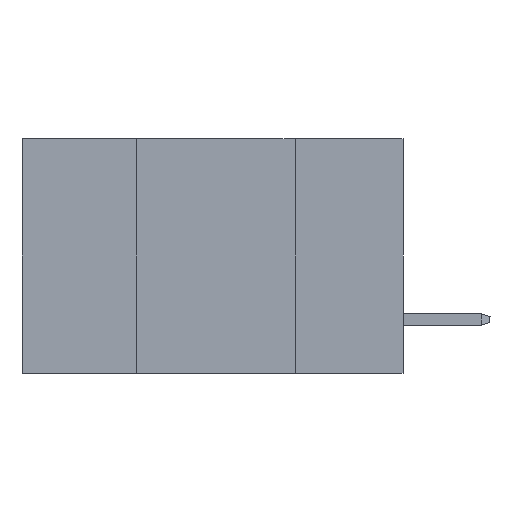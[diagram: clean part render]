
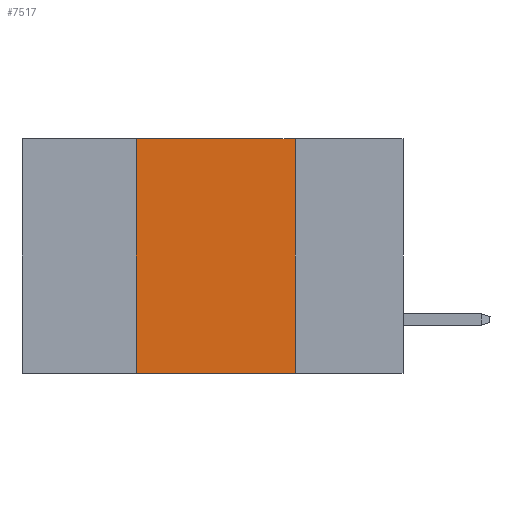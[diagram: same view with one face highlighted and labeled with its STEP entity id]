
A CAD part, left-side view. The second image highlights one B-rep face of the part: STEP entity #7517.
In plain terms, the highlighted planar face has unit normal (-1, 0, 0).
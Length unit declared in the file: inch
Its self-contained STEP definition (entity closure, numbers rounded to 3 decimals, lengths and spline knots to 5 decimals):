
#582 = CARTESIAN_POINT ( 'NONE',  ( 0., 0.6, 0. ) ) ;
#982 = LINE ( 'NONE', #5002, #21636 ) ;
#1261 = CARTESIAN_POINT ( 'NONE',  ( 0., 0.17, 0. ) ) ;
#1351 = VERTEX_POINT ( 'NONE', #9151 ) ;
#1695 = AXIS2_PLACEMENT_3D ( 'NONE', #582, #12738, #18744 ) ;
#3512 = ORIENTED_EDGE ( 'NONE', *, *, #24849, .T. ) ;
#4922 = LINE ( 'NONE', #15397, #11618 ) ;
#5002 = CARTESIAN_POINT ( 'NONE',  ( 0., 0.42, 0. ) ) ;
#6378 = VERTEX_POINT ( 'NONE', #22240 ) ;
#7517 = ADVANCED_FACE ( 'NONE', ( #20680 ), #22874, .F. ) ;
#8569 = EDGE_LOOP ( 'NONE', ( #20301, #10029, #10671, #3512 ) ) ;
#9151 = CARTESIAN_POINT ( 'NONE',  ( 0., 0.42, -0.37 ) ) ;
#10029 = ORIENTED_EDGE ( 'NONE', *, *, #14172, .F. ) ;
#10671 = ORIENTED_EDGE ( 'NONE', *, *, #16047, .F. ) ;
#11433 = VECTOR ( 'NONE', #15040, 39.37008 ) ;
#11618 = VECTOR ( 'NONE', #16856, 39.37008 ) ;
#12738 = DIRECTION ( 'NONE',  ( 1., 0., 0. ) ) ;
#14172 = EDGE_CURVE ( 'NONE', #17488, #18652, #4922, .T. ) ;
#14842 = DIRECTION ( 'NONE',  ( 0., 0., 1. ) ) ;
#15040 = DIRECTION ( 'NONE',  ( 0., -1., 0. ) ) ;
#15372 = DIRECTION ( 'NONE',  ( 0., 0., -1. ) ) ;
#15397 = CARTESIAN_POINT ( 'NONE',  ( 0., 0.6, 0. ) ) ;
#15503 = LINE ( 'NONE', #1261, #20932 ) ;
#16047 = EDGE_CURVE ( 'NONE', #1351, #17488, #982, .T. ) ;
#16856 = DIRECTION ( 'NONE',  ( 0., -1., 0. ) ) ;
#17135 = LINE ( 'NONE', #20894, #11433 ) ;
#17488 = VERTEX_POINT ( 'NONE', #23311 ) ;
#18652 = VERTEX_POINT ( 'NONE', #20739 ) ;
#18744 = DIRECTION ( 'NONE',  ( 0., 0., -1. ) ) ;
#20301 = ORIENTED_EDGE ( 'NONE', *, *, #20471, .F. ) ;
#20471 = EDGE_CURVE ( 'NONE', #18652, #6378, #15503, .T. ) ;
#20680 = FACE_OUTER_BOUND ( 'NONE', #8569, .T. ) ;
#20739 = CARTESIAN_POINT ( 'NONE',  ( 0., 0.17, 0. ) ) ;
#20894 = CARTESIAN_POINT ( 'NONE',  ( 0., 0.6, -0.37 ) ) ;
#20932 = VECTOR ( 'NONE', #15372, 39.37008 ) ;
#21636 = VECTOR ( 'NONE', #14842, 39.37008 ) ;
#22240 = CARTESIAN_POINT ( 'NONE',  ( 0., 0.17, -0.37 ) ) ;
#22874 = PLANE ( 'NONE',  #1695 ) ;
#23311 = CARTESIAN_POINT ( 'NONE',  ( 0., 0.42, 0. ) ) ;
#24849 = EDGE_CURVE ( 'NONE', #1351, #6378, #17135, .T. ) ;
